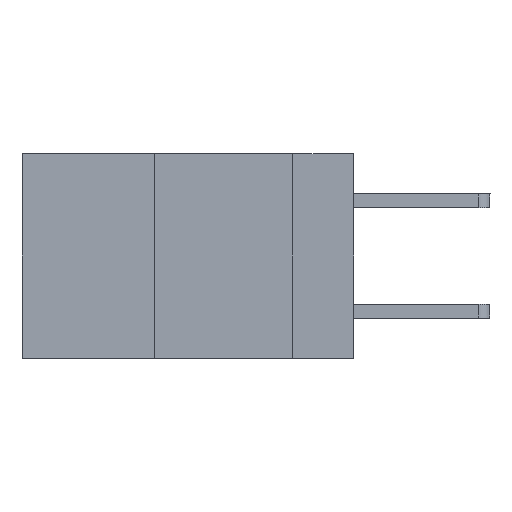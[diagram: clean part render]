
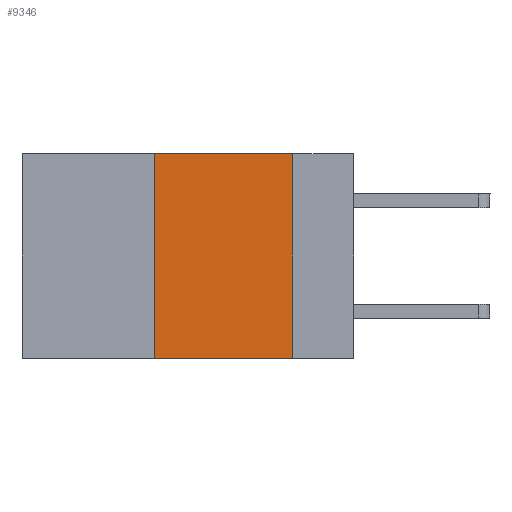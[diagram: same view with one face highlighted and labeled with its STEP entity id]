
A CAD part, left-side view. The second image highlights one B-rep face of the part: STEP entity #9346.
In plain terms, the highlighted planar face has unit normal (-1, 0, 0).
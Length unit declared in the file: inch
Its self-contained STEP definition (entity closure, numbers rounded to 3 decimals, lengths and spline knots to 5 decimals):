
#80 = CARTESIAN_POINT ( 'NONE',  ( 0., 0.11, 0. ) ) ;
#689 = VERTEX_POINT ( 'NONE', #2157 ) ;
#771 = DIRECTION ( 'NONE',  ( 0., 0., -1. ) ) ;
#1553 = ORIENTED_EDGE ( 'NONE', *, *, #11956, .T. ) ;
#1669 = CARTESIAN_POINT ( 'NONE',  ( 0., 0.6, -0.37 ) ) ;
#1736 = FACE_OUTER_BOUND ( 'NONE', #5180, .T. ) ;
#1957 = AXIS2_PLACEMENT_3D ( 'NONE', #12623, #10764, #771 ) ;
#2139 = ORIENTED_EDGE ( 'NONE', *, *, #12118, .F. ) ;
#2157 = CARTESIAN_POINT ( 'NONE',  ( 0., 0.36, -0.37 ) ) ;
#2472 = VECTOR ( 'NONE', #11020, 39.37008 ) ;
#2906 = PLANE ( 'NONE',  #1957 ) ;
#2916 = VERTEX_POINT ( 'NONE', #3558 ) ;
#3108 = LINE ( 'NONE', #1669, #10627 ) ;
#3558 = CARTESIAN_POINT ( 'NONE',  ( 0., 0.11, -0.37 ) ) ;
#3877 = EDGE_CURVE ( 'NONE', #689, #4072, #11167, .T. ) ;
#4072 = VERTEX_POINT ( 'NONE', #6133 ) ;
#4643 = DIRECTION ( 'NONE',  ( 0., -1., 0. ) ) ;
#5180 = EDGE_LOOP ( 'NONE', ( #2139, #8170, #5883, #1553 ) ) ;
#5312 = LINE ( 'NONE', #7096, #6390 ) ;
#5645 = CARTESIAN_POINT ( 'NONE',  ( 0., 0.36, 0. ) ) ;
#5883 = ORIENTED_EDGE ( 'NONE', *, *, #3877, .F. ) ;
#6133 = CARTESIAN_POINT ( 'NONE',  ( 0., 0.36, 0. ) ) ;
#6390 = VECTOR ( 'NONE', #11188, 39.37008 ) ;
#6792 = DIRECTION ( 'NONE',  ( 0., 0., 1. ) ) ;
#7096 = CARTESIAN_POINT ( 'NONE',  ( 0., 0.6, 0. ) ) ;
#7639 = EDGE_CURVE ( 'NONE', #4072, #8849, #5312, .T. ) ;
#8170 = ORIENTED_EDGE ( 'NONE', *, *, #7639, .F. ) ;
#8849 = VERTEX_POINT ( 'NONE', #9838 ) ;
#9346 = ADVANCED_FACE ( 'NONE', ( #1736 ), #2906, .F. ) ;
#9562 = LINE ( 'NONE', #80, #2472 ) ;
#9838 = CARTESIAN_POINT ( 'NONE',  ( 0., 0.11, 0. ) ) ;
#10627 = VECTOR ( 'NONE', #4643, 39.37008 ) ;
#10764 = DIRECTION ( 'NONE',  ( 1., 0., 0. ) ) ;
#10919 = VECTOR ( 'NONE', #6792, 39.37008 ) ;
#11020 = DIRECTION ( 'NONE',  ( 0., 0., -1. ) ) ;
#11167 = LINE ( 'NONE', #5645, #10919 ) ;
#11188 = DIRECTION ( 'NONE',  ( 0., -1., 0. ) ) ;
#11956 = EDGE_CURVE ( 'NONE', #689, #2916, #3108, .T. ) ;
#12118 = EDGE_CURVE ( 'NONE', #8849, #2916, #9562, .T. ) ;
#12623 = CARTESIAN_POINT ( 'NONE',  ( 0., 0.6, 0. ) ) ;
